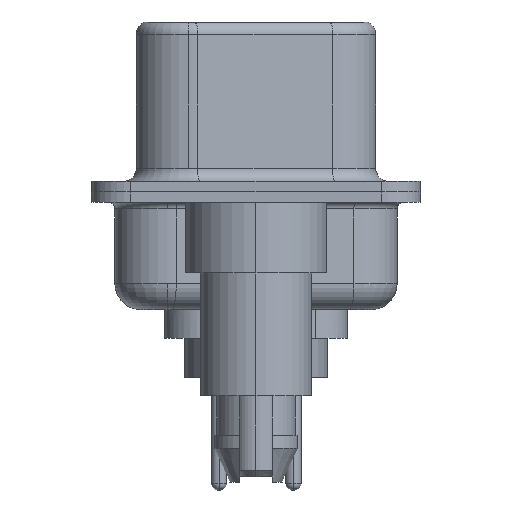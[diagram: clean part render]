
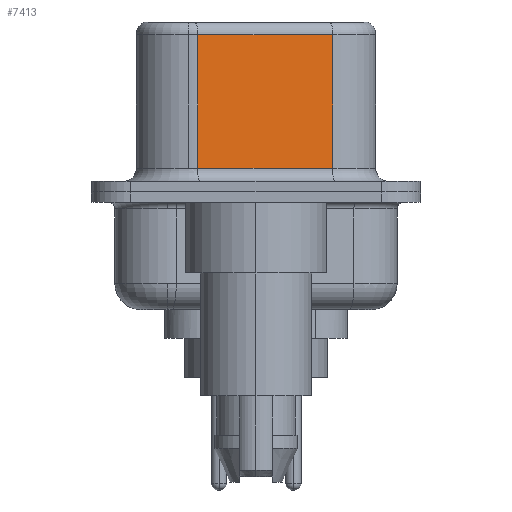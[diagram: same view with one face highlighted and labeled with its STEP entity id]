
A CAD part, left-side view. The second image highlights one B-rep face of the part: STEP entity #7413.
In plain terms, the highlighted planar face has unit normal (-0.985, -0.174, 0).
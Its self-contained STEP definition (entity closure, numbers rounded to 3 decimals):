
#1511 = CARTESIAN_POINT ( 'NONE',  ( 4.585, -2.927, 6.52 ) ) ;
#2931 = DIRECTION ( 'NONE',  ( 0., 0., -1. ) ) ;
#2999 = ORIENTED_EDGE ( 'NONE', *, *, #11971, .T. ) ;
#3021 = VERTEX_POINT ( 'NONE', #4591 ) ;
#3129 = AXIS2_PLACEMENT_3D ( 'NONE', #13799, #15256, #6804 ) ;
#3584 = DIRECTION ( 'NONE',  ( -0.174, 0.985, 0. ) ) ;
#3902 = PLANE ( 'NONE',  #3129 ) ;
#3922 = LINE ( 'NONE', #11107, #17810 ) ;
#4591 = CARTESIAN_POINT ( 'NONE',  ( 4.585, -2.927, 6.02 ) ) ;
#5543 = DIRECTION ( 'NONE',  ( 0.174, -0.985, 0. ) ) ;
#5892 = VECTOR ( 'NONE', #2931, 1000. ) ;
#6678 = VERTEX_POINT ( 'NONE', #16912 ) ;
#6804 = DIRECTION ( 'NONE',  ( -0.174, 0.985, 0. ) ) ;
#7157 = DIRECTION ( 'NONE',  ( 0., 0., -1. ) ) ;
#7212 = ORIENTED_EDGE ( 'NONE', *, *, #13529, .F. ) ;
#7413 = ADVANCED_FACE ( 'NONE', ( #11520 ), #3902, .F. ) ;
#10035 = ORIENTED_EDGE ( 'NONE', *, *, #13477, .T. ) ;
#10300 = VERTEX_POINT ( 'NONE', #10790 ) ;
#10541 = EDGE_CURVE ( 'NONE', #6678, #10300, #14704, .T. ) ;
#10790 = CARTESIAN_POINT ( 'NONE',  ( 3.675, 2.233, 0.9 ) ) ;
#10858 = VECTOR ( 'NONE', #7157, 1000. ) ;
#11107 = CARTESIAN_POINT ( 'NONE',  ( 4.585, -2.927, 0.9 ) ) ;
#11240 = CARTESIAN_POINT ( 'NONE',  ( 3.675, 2.233, 6.52 ) ) ;
#11520 = FACE_OUTER_BOUND ( 'NONE', #14537, .T. ) ;
#11971 = EDGE_CURVE ( 'NONE', #3021, #6678, #14168, .T. ) ;
#13476 = CARTESIAN_POINT ( 'NONE',  ( 4.585, -2.927, 6.02 ) ) ;
#13477 = EDGE_CURVE ( 'NONE', #10300, #15014, #3922, .T. ) ;
#13529 = EDGE_CURVE ( 'NONE', #3021, #15014, #17010, .T. ) ;
#13733 = VECTOR ( 'NONE', #3584, 1000. ) ;
#13799 = CARTESIAN_POINT ( 'NONE',  ( 4.585, -2.927, 6.52 ) ) ;
#13822 = ORIENTED_EDGE ( 'NONE', *, *, #10541, .T. ) ;
#14168 = LINE ( 'NONE', #13476, #13733 ) ;
#14537 = EDGE_LOOP ( 'NONE', ( #7212, #2999, #13822, #10035 ) ) ;
#14704 = LINE ( 'NONE', #11240, #10858 ) ;
#15014 = VERTEX_POINT ( 'NONE', #15170 ) ;
#15170 = CARTESIAN_POINT ( 'NONE',  ( 4.585, -2.927, 0.9 ) ) ;
#15256 = DIRECTION ( 'NONE',  ( 0.985, 0.174, 0. ) ) ;
#16912 = CARTESIAN_POINT ( 'NONE',  ( 3.675, 2.233, 6.02 ) ) ;
#17010 = LINE ( 'NONE', #1511, #5892 ) ;
#17810 = VECTOR ( 'NONE', #5543, 1000. ) ;
